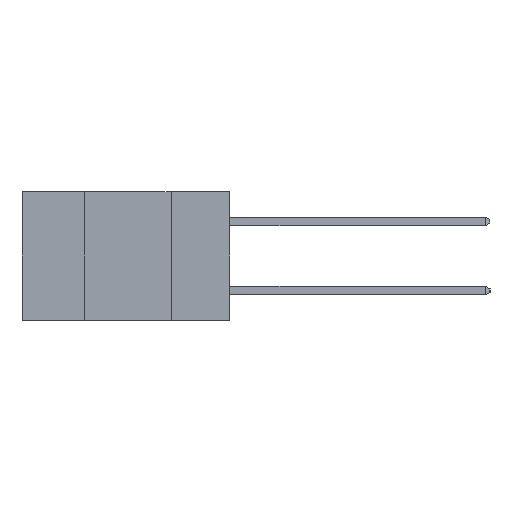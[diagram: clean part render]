
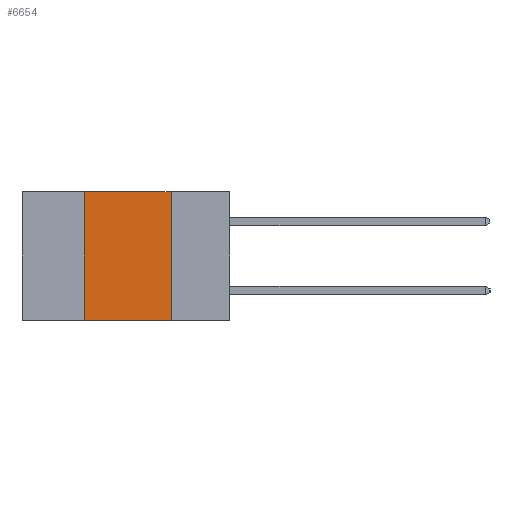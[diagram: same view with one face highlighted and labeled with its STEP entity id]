
A CAD part, left-side view. The second image highlights one B-rep face of the part: STEP entity #6654.
In plain terms, the highlighted planar face has unit normal (-1, 0, 0).
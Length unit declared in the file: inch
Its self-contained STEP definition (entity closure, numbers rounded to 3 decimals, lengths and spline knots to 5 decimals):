
#244 = ORIENTED_EDGE ( 'NONE', *, *, #10998, .F. ) ;
#251 = LINE ( 'NONE', #3078, #10818 ) ;
#404 = AXIS2_PLACEMENT_3D ( 'NONE', #8658, #8617, #8615 ) ;
#1172 = VECTOR ( 'NONE', #2199, 39.37008 ) ;
#2199 = DIRECTION ( 'NONE',  ( 0., 0., -1. ) ) ;
#2348 = ORIENTED_EDGE ( 'NONE', *, *, #3230, .T. ) ;
#2533 = EDGE_CURVE ( 'NONE', #7624, #5522, #4045, .T. ) ;
#2963 = VERTEX_POINT ( 'NONE', #12444 ) ;
#3078 = CARTESIAN_POINT ( 'NONE',  ( 0., 0.6, 0. ) ) ;
#3230 = EDGE_CURVE ( 'NONE', #7624, #9975, #10889, .T. ) ;
#3665 = DIRECTION ( 'NONE',  ( 0., -1., 0. ) ) ;
#3728 = VECTOR ( 'NONE', #9279, 39.37008 ) ;
#3944 = CARTESIAN_POINT ( 'NONE',  ( 0., 0.17, -0.37 ) ) ;
#3947 = CARTESIAN_POINT ( 'NONE',  ( 0., 0.42, 0. ) ) ;
#3964 = CARTESIAN_POINT ( 'NONE',  ( 0., 0.42, -0.37 ) ) ;
#4045 = LINE ( 'NONE', #9346, #3728 ) ;
#4535 = LINE ( 'NONE', #3944, #1172 ) ;
#5454 = VECTOR ( 'NONE', #10505, 39.37008 ) ;
#5522 = VERTEX_POINT ( 'NONE', #3947 ) ;
#5696 = ORIENTED_EDGE ( 'NONE', *, *, #9697, .F. ) ;
#6583 = EDGE_LOOP ( 'NONE', ( #244, #5696, #6681, #2348 ) ) ;
#6654 = ADVANCED_FACE ( 'NONE', ( #12552 ), #8646, .F. ) ;
#6681 = ORIENTED_EDGE ( 'NONE', *, *, #2533, .F. ) ;
#7624 = VERTEX_POINT ( 'NONE', #3964 ) ;
#8582 = CARTESIAN_POINT ( 'NONE',  ( 0., 0.17, -0.37 ) ) ;
#8615 = DIRECTION ( 'NONE',  ( 0., 0., -1. ) ) ;
#8617 = DIRECTION ( 'NONE',  ( 1., 0., 0. ) ) ;
#8646 = PLANE ( 'NONE',  #404 ) ;
#8658 = CARTESIAN_POINT ( 'NONE',  ( 0., 0.6, 0. ) ) ;
#9279 = DIRECTION ( 'NONE',  ( 0., 0., 1. ) ) ;
#9346 = CARTESIAN_POINT ( 'NONE',  ( 0., 0.42, -0.37 ) ) ;
#9697 = EDGE_CURVE ( 'NONE', #5522, #2963, #251, .T. ) ;
#9975 = VERTEX_POINT ( 'NONE', #8582 ) ;
#10505 = DIRECTION ( 'NONE',  ( 0., -1., 0. ) ) ;
#10536 = CARTESIAN_POINT ( 'NONE',  ( 0., 0.6, -0.37 ) ) ;
#10818 = VECTOR ( 'NONE', #3665, 39.37008 ) ;
#10889 = LINE ( 'NONE', #10536, #5454 ) ;
#10998 = EDGE_CURVE ( 'NONE', #2963, #9975, #4535, .T. ) ;
#12444 = CARTESIAN_POINT ( 'NONE',  ( 0., 0.17, 0. ) ) ;
#12552 = FACE_OUTER_BOUND ( 'NONE', #6583, .T. ) ;
